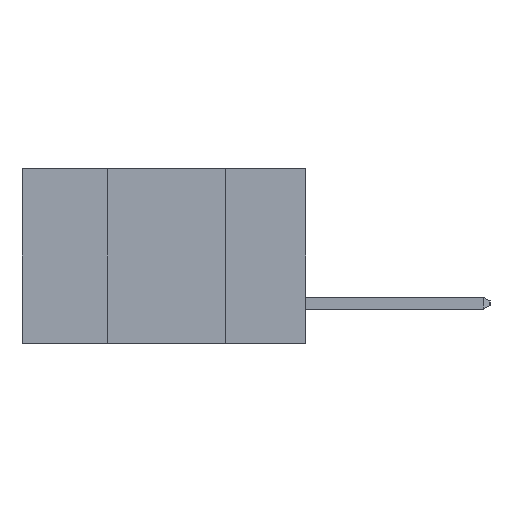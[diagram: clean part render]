
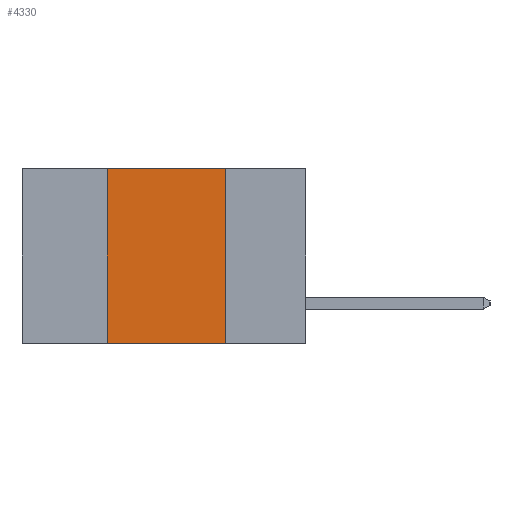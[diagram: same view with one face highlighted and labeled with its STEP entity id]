
A CAD part, left-side view. The second image highlights one B-rep face of the part: STEP entity #4330.
In plain terms, the highlighted planar face has unit normal (-1, 0, 0).
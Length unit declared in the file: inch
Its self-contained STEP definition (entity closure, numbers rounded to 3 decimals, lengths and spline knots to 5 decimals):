
#844 = EDGE_CURVE ( 'NONE', #2917, #18073, #15907, .T. ) ;
#2436 = CARTESIAN_POINT ( 'NONE',  ( 0., 0.17, 0. ) ) ;
#2855 = ORIENTED_EDGE ( 'NONE', *, *, #844, .F. ) ;
#2917 = VERTEX_POINT ( 'NONE', #17506 ) ;
#3289 = ORIENTED_EDGE ( 'NONE', *, *, #4318, .F. ) ;
#4120 = VERTEX_POINT ( 'NONE', #21976 ) ;
#4318 = EDGE_CURVE ( 'NONE', #18073, #17460, #13580, .T. ) ;
#4330 = ADVANCED_FACE ( 'NONE', ( #21421 ), #15578, .F. ) ;
#4477 = ORIENTED_EDGE ( 'NONE', *, *, #10133, .T. ) ;
#6589 = EDGE_LOOP ( 'NONE', ( #16097, #3289, #2855, #4477 ) ) ;
#7606 = CARTESIAN_POINT ( 'NONE',  ( 0., 0.6, -0.37 ) ) ;
#7843 = DIRECTION ( 'NONE',  ( 0., -1., 0. ) ) ;
#7965 = CARTESIAN_POINT ( 'NONE',  ( 0., 0.6, 0. ) ) ;
#8058 = DIRECTION ( 'NONE',  ( 1., 0., 0. ) ) ;
#8514 = DIRECTION ( 'NONE',  ( 0., 0., -1. ) ) ;
#9630 = VECTOR ( 'NONE', #16603, 39.37008 ) ;
#10133 = EDGE_CURVE ( 'NONE', #2917, #4120, #12187, .T. ) ;
#11111 = VECTOR ( 'NONE', #7843, 39.37008 ) ;
#12187 = LINE ( 'NONE', #7606, #11111 ) ;
#12217 = CARTESIAN_POINT ( 'NONE',  ( 0., 0.17, -0.37 ) ) ;
#13580 = LINE ( 'NONE', #15682, #9630 ) ;
#14462 = CARTESIAN_POINT ( 'NONE',  ( 0., 0.42, 0. ) ) ;
#14786 = VECTOR ( 'NONE', #20583, 39.37008 ) ;
#15578 = PLANE ( 'NONE',  #17225 ) ;
#15641 = CARTESIAN_POINT ( 'NONE',  ( 0., 0.42, -0.37 ) ) ;
#15682 = CARTESIAN_POINT ( 'NONE',  ( 0., 0.6, 0. ) ) ;
#15907 = LINE ( 'NONE', #15641, #19808 ) ;
#16097 = ORIENTED_EDGE ( 'NONE', *, *, #18502, .F. ) ;
#16603 = DIRECTION ( 'NONE',  ( 0., -1., 0. ) ) ;
#17225 = AXIS2_PLACEMENT_3D ( 'NONE', #7965, #8058, #8514 ) ;
#17460 = VERTEX_POINT ( 'NONE', #2436 ) ;
#17506 = CARTESIAN_POINT ( 'NONE',  ( 0., 0.42, -0.37 ) ) ;
#18073 = VERTEX_POINT ( 'NONE', #14462 ) ;
#18502 = EDGE_CURVE ( 'NONE', #17460, #4120, #19781, .T. ) ;
#18936 = DIRECTION ( 'NONE',  ( 0., 0., 1. ) ) ;
#19781 = LINE ( 'NONE', #12217, #14786 ) ;
#19808 = VECTOR ( 'NONE', #18936, 39.37008 ) ;
#20583 = DIRECTION ( 'NONE',  ( 0., 0., -1. ) ) ;
#21421 = FACE_OUTER_BOUND ( 'NONE', #6589, .T. ) ;
#21976 = CARTESIAN_POINT ( 'NONE',  ( 0., 0.17, -0.37 ) ) ;
